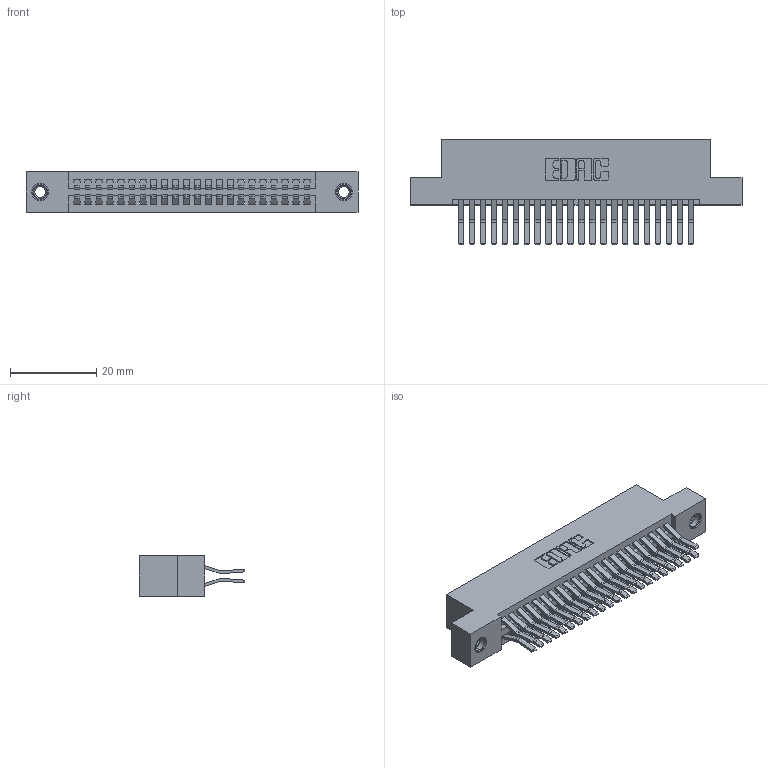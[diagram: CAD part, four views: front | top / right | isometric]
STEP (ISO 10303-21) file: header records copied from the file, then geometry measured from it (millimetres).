
FILE_DESCRIPTION (( 'STEP AP203' ), '1' );
FILE_NAME ('395-044-560-207.STEP', '2019-10-19T03:14:48', ( '' ), ( '' ), 'SwSTEP 2.0', 'SolidWorks 2016', '' );
FILE_SCHEMA (( 'CONFIG_CONTROL_DESIGN' ));
Length unit declared in the file: inch
Products named in the file (4): 395-044-560-207; 345 Part_Flush Mounting Lugs - 0.156 Dia-TI; 345-292-001_560 Tail; 345-250-001_345-250-005-103
Assembly tree (47 placements, depth 2):
  395-044-560-207
    345 Part_Flush Mounting Lugs - 0.156 Dia-TI
    345-292-001_560 Tail  x44
    345-250-001_345-250-005-103  x2
Bounding box: 77.09 x 24.45 x 9.4 mm (x, y, z)
Volume: 7577.7 mm3; surface area: 11583.4 mm2
Topology: 47 solids, 47 shells, 2474 faces, 7297 edges, 4798 vertices
Faces by surface type: plane 1564, cylinder 894, cone 12, torus 4
Entity records: 21228 total; most frequent: CARTESIAN_POINT 3559, ORIENTED_EDGE 3486, DIRECTION 3193, EDGE_CURVE 1743, LINE 1499, VECTOR 1499, VERTEX_POINT 1156, AXIS2_PLACEMENT_3D 847
